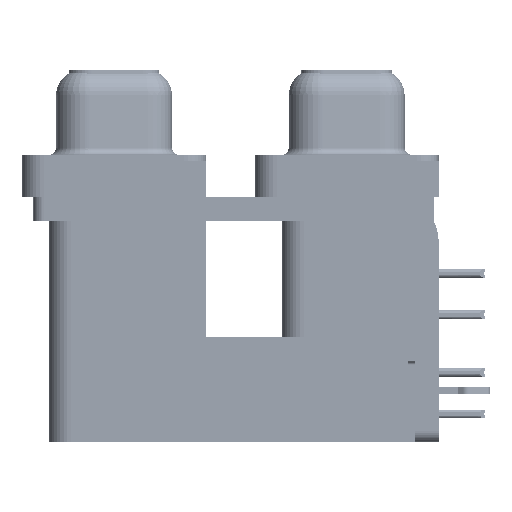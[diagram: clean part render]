
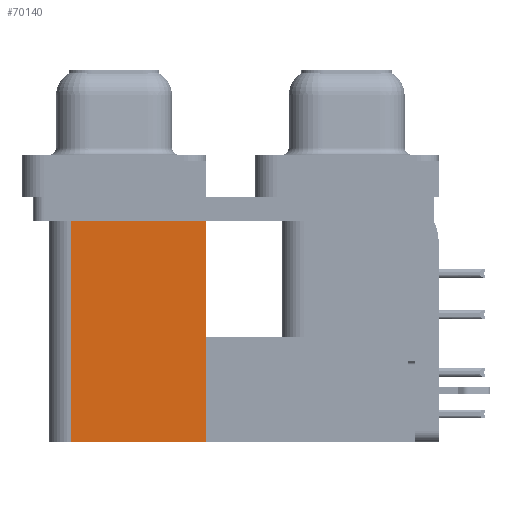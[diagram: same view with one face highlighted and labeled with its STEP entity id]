
A CAD part, left-side view. The second image highlights one B-rep face of the part: STEP entity #70140.
In plain terms, the highlighted planar face has unit normal (-1, 0, 0).
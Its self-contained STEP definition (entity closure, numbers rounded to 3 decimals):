
#110 = ORIENTED_EDGE ( 'NONE', *, *, #31648, .T. ) ;
#799 = CARTESIAN_POINT ( 'NONE',  ( 3.79, 9.6, -19.2 ) ) ;
#5610 = LINE ( 'NONE', #38858, #58020 ) ;
#11154 = DIRECTION ( 'NONE',  ( 0., 0., -1. ) ) ;
#12420 = DIRECTION ( 'NONE',  ( 0., 1., 0. ) ) ;
#14062 = CARTESIAN_POINT ( 'NONE',  ( 3.79, 9.6, -2.5 ) ) ;
#14745 = DIRECTION ( 'NONE',  ( 0., 1., 0. ) ) ;
#17960 = EDGE_CURVE ( 'NONE', #51620, #31277, #5610, .T. ) ;
#18904 = EDGE_CURVE ( 'NONE', #60874, #51620, #40818, .T. ) ;
#21444 = CARTESIAN_POINT ( 'NONE',  ( 3.79, 9.6, -2.5 ) ) ;
#23502 = CARTESIAN_POINT ( 'NONE',  ( 3.79, 9.6, -19.2 ) ) ;
#28418 = DIRECTION ( 'NONE',  ( 0., 0., 1. ) ) ;
#28854 = DIRECTION ( 'NONE',  ( 0., 0., 1. ) ) ;
#31277 = VERTEX_POINT ( 'NONE', #72321 ) ;
#31648 = EDGE_CURVE ( 'NONE', #60874, #38345, #40783, .T. ) ;
#33944 = PLANE ( 'NONE',  #42261 ) ;
#38345 = VERTEX_POINT ( 'NONE', #14062 ) ;
#38858 = CARTESIAN_POINT ( 'NONE',  ( 3.79, 18.8, -19.2 ) ) ;
#40783 = LINE ( 'NONE', #799, #62772 ) ;
#40818 = LINE ( 'NONE', #63642, #71248 ) ;
#42261 = AXIS2_PLACEMENT_3D ( 'NONE', #23502, #57524, #11154 ) ;
#45160 = FACE_OUTER_BOUND ( 'NONE', #64740, .T. ) ;
#51620 = VERTEX_POINT ( 'NONE', #67717 ) ;
#55647 = ORIENTED_EDGE ( 'NONE', *, *, #18904, .F. ) ;
#57524 = DIRECTION ( 'NONE',  ( 1., 0., 0. ) ) ;
#58020 = VECTOR ( 'NONE', #28418, 1000. ) ;
#58791 = CARTESIAN_POINT ( 'NONE',  ( 3.79, 9.6, -19.2 ) ) ;
#60874 = VERTEX_POINT ( 'NONE', #58791 ) ;
#62772 = VECTOR ( 'NONE', #28854, 1000. ) ;
#63642 = CARTESIAN_POINT ( 'NONE',  ( 3.79, 9.6, -19.2 ) ) ;
#64071 = VECTOR ( 'NONE', #14745, 1000. ) ;
#64243 = ORIENTED_EDGE ( 'NONE', *, *, #65853, .T. ) ;
#64740 = EDGE_LOOP ( 'NONE', ( #64243, #73438, #55647, #110 ) ) ;
#65853 = EDGE_CURVE ( 'NONE', #38345, #31277, #65956, .T. ) ;
#65956 = LINE ( 'NONE', #21444, #64071 ) ;
#67717 = CARTESIAN_POINT ( 'NONE',  ( 3.79, 18.8, -19.2 ) ) ;
#70140 = ADVANCED_FACE ( 'NONE', ( #45160 ), #33944, .F. ) ;
#71248 = VECTOR ( 'NONE', #12420, 1000. ) ;
#72321 = CARTESIAN_POINT ( 'NONE',  ( 3.79, 18.8, -2.5 ) ) ;
#73438 = ORIENTED_EDGE ( 'NONE', *, *, #17960, .F. ) ;
